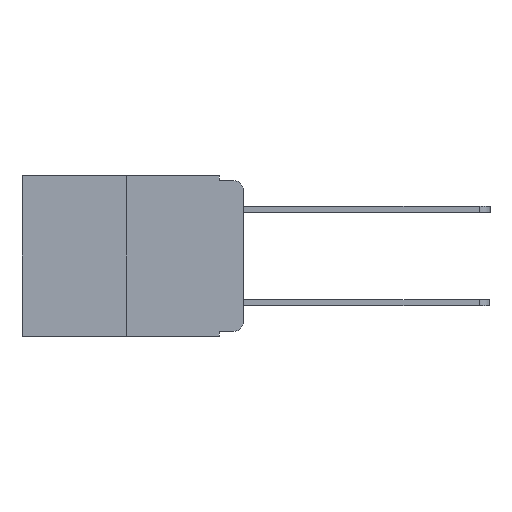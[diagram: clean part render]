
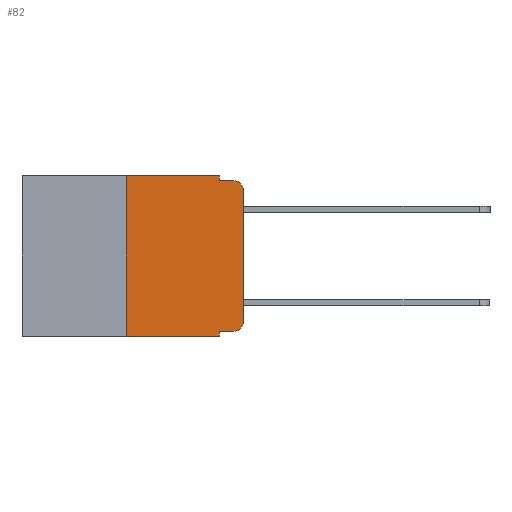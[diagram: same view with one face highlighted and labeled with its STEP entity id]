
A CAD part, left-side view. The second image highlights one B-rep face of the part: STEP entity #82.
In plain terms, the highlighted planar face has unit normal (-1, 0, 0).
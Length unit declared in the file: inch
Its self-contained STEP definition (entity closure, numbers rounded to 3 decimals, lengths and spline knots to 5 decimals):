
#37 = DIRECTION ( 'NONE',  ( 0., -1., 0. ) ) ;
#82 = ADVANCED_FACE ( 'NONE', ( #8506 ), #4938, .F. ) ;
#83 = ORIENTED_EDGE ( 'NONE', *, *, #11545, .F. ) ;
#535 = VECTOR ( 'NONE', #12441, 39.37008 ) ;
#607 = CARTESIAN_POINT ( 'NONE',  ( 0., 0.051, 0. ) ) ;
#692 = ORIENTED_EDGE ( 'NONE', *, *, #1573, .T. ) ;
#735 = VERTEX_POINT ( 'NONE', #11235 ) ;
#830 = VECTOR ( 'NONE', #37, 39.37008 ) ;
#973 = DIRECTION ( 'NONE',  ( 0., 0., 1. ) ) ;
#1096 = CARTESIAN_POINT ( 'NONE',  ( 0., 0.25, -0.343 ) ) ;
#1404 = VECTOR ( 'NONE', #973, 39.37008 ) ;
#1506 = CIRCLE ( 'NONE', #15922, 0.02 ) ;
#1526 = ORIENTED_EDGE ( 'NONE', *, *, #14871, .F. ) ;
#1573 = EDGE_CURVE ( 'NONE', #7231, #10389, #1824, .T. ) ;
#1706 = CARTESIAN_POINT ( 'NONE',  ( 0., 0.25, 0. ) ) ;
#1824 = LINE ( 'NONE', #13925, #1404 ) ;
#2142 = VERTEX_POINT ( 'NONE', #14864 ) ;
#2249 = AXIS2_PLACEMENT_3D ( 'NONE', #2256, #11621, #10146 ) ;
#2256 = CARTESIAN_POINT ( 'NONE',  ( 0., 0.473, 0. ) ) ;
#2350 = CARTESIAN_POINT ( 'NONE',  ( 0., 0.051, 0. ) ) ;
#2392 = ORIENTED_EDGE ( 'NONE', *, *, #12402, .F. ) ;
#2528 = CARTESIAN_POINT ( 'NONE',  ( 0., 0.051, -0.343 ) ) ;
#2673 = VERTEX_POINT ( 'NONE', #1706 ) ;
#2821 = CARTESIAN_POINT ( 'NONE',  ( 0., 0.02, -0.03 ) ) ;
#3191 = EDGE_LOOP ( 'NONE', ( #692, #4683, #1526, #15228, #8986, #2392, #9764, #83, #10808, #7807 ) ) ;
#3380 = DIRECTION ( 'NONE',  ( 0., 0., -1. ) ) ;
#3382 = CARTESIAN_POINT ( 'NONE',  ( 0., 0.051, -0.01 ) ) ;
#3388 = VERTEX_POINT ( 'NONE', #4537 ) ;
#3515 = VECTOR ( 'NONE', #12458, 39.37008 ) ;
#3528 = LINE ( 'NONE', #14906, #13782 ) ;
#3818 = VERTEX_POINT ( 'NONE', #2528 ) ;
#4020 = LINE ( 'NONE', #14276, #830 ) ;
#4168 = DIRECTION ( 'NONE',  ( 0., 0., -1. ) ) ;
#4192 = DIRECTION ( 'NONE',  ( -1., 0., 0. ) ) ;
#4537 = CARTESIAN_POINT ( 'NONE',  ( 0., 0.02, -0.01 ) ) ;
#4683 = ORIENTED_EDGE ( 'NONE', *, *, #16473, .T. ) ;
#4741 = EDGE_CURVE ( 'NONE', #16317, #3818, #4020, .T. ) ;
#4938 = PLANE ( 'NONE',  #2249 ) ;
#5110 = CARTESIAN_POINT ( 'NONE',  ( 0., 0.051, -0.333 ) ) ;
#6439 = DIRECTION ( 'NONE',  ( 0., -1., 0. ) ) ;
#6491 = CARTESIAN_POINT ( 'NONE',  ( 0., 0.02, -0.333 ) ) ;
#6987 = VECTOR ( 'NONE', #6439, 39.37008 ) ;
#7014 = LINE ( 'NONE', #14879, #3515 ) ;
#7197 = LINE ( 'NONE', #3382, #535 ) ;
#7231 = VERTEX_POINT ( 'NONE', #12112 ) ;
#7807 = ORIENTED_EDGE ( 'NONE', *, *, #8123, .T. ) ;
#7869 = VECTOR ( 'NONE', #9498, 39.37008 ) ;
#8123 = EDGE_CURVE ( 'NONE', #15779, #7231, #10787, .T. ) ;
#8208 = CARTESIAN_POINT ( 'NONE',  ( 0., 0.25, 0. ) ) ;
#8281 = LINE ( 'NONE', #8208, #7869 ) ;
#8506 = FACE_OUTER_BOUND ( 'NONE', #3191, .T. ) ;
#8986 = ORIENTED_EDGE ( 'NONE', *, *, #14219, .F. ) ;
#9175 = AXIS2_PLACEMENT_3D ( 'NONE', #11917, #4192, #13191 ) ;
#9498 = DIRECTION ( 'NONE',  ( 0., 0., 1. ) ) ;
#9677 = VERTEX_POINT ( 'NONE', #607 ) ;
#9764 = ORIENTED_EDGE ( 'NONE', *, *, #4741, .T. ) ;
#9832 = EDGE_CURVE ( 'NONE', #2142, #15779, #13749, .T. ) ;
#10146 = DIRECTION ( 'NONE',  ( 0., 0., -1. ) ) ;
#10389 = VERTEX_POINT ( 'NONE', #15411 ) ;
#10787 = CIRCLE ( 'NONE', #9175, 0.02 ) ;
#10808 = ORIENTED_EDGE ( 'NONE', *, *, #9832, .T. ) ;
#11235 = CARTESIAN_POINT ( 'NONE',  ( 0., 0.051, -0.01 ) ) ;
#11458 = DIRECTION ( 'NONE',  ( 0., 0., -1. ) ) ;
#11545 = EDGE_CURVE ( 'NONE', #2142, #3818, #11697, .T. ) ;
#11621 = DIRECTION ( 'NONE',  ( 1., 0., 0. ) ) ;
#11697 = LINE ( 'NONE', #2350, #14979 ) ;
#11896 = DIRECTION ( 'NONE',  ( -1., 0., 0. ) ) ;
#11917 = CARTESIAN_POINT ( 'NONE',  ( 0., 0.02, -0.313 ) ) ;
#12112 = CARTESIAN_POINT ( 'NONE',  ( 0., 0., -0.313 ) ) ;
#12402 = EDGE_CURVE ( 'NONE', #16317, #2673, #8281, .T. ) ;
#12441 = DIRECTION ( 'NONE',  ( 0., -1., 0. ) ) ;
#12458 = DIRECTION ( 'NONE',  ( 0., -1., 0. ) ) ;
#13191 = DIRECTION ( 'NONE',  ( 0., 0., -1. ) ) ;
#13237 = EDGE_CURVE ( 'NONE', #9677, #735, #3528, .T. ) ;
#13749 = LINE ( 'NONE', #5110, #6987 ) ;
#13782 = VECTOR ( 'NONE', #3380, 39.37008 ) ;
#13925 = CARTESIAN_POINT ( 'NONE',  ( 0., 0., 0. ) ) ;
#14219 = EDGE_CURVE ( 'NONE', #2673, #9677, #7014, .T. ) ;
#14276 = CARTESIAN_POINT ( 'NONE',  ( 0., 0.473, -0.343 ) ) ;
#14864 = CARTESIAN_POINT ( 'NONE',  ( 0., 0.051, -0.333 ) ) ;
#14871 = EDGE_CURVE ( 'NONE', #735, #3388, #7197, .T. ) ;
#14879 = CARTESIAN_POINT ( 'NONE',  ( 0., 0.473, 0. ) ) ;
#14906 = CARTESIAN_POINT ( 'NONE',  ( 0., 0.051, 0. ) ) ;
#14979 = VECTOR ( 'NONE', #11458, 39.37008 ) ;
#15228 = ORIENTED_EDGE ( 'NONE', *, *, #13237, .F. ) ;
#15411 = CARTESIAN_POINT ( 'NONE',  ( 0., 0., -0.03 ) ) ;
#15779 = VERTEX_POINT ( 'NONE', #6491 ) ;
#15922 = AXIS2_PLACEMENT_3D ( 'NONE', #2821, #11896, #4168 ) ;
#16317 = VERTEX_POINT ( 'NONE', #1096 ) ;
#16473 = EDGE_CURVE ( 'NONE', #10389, #3388, #1506, .T. ) ;
